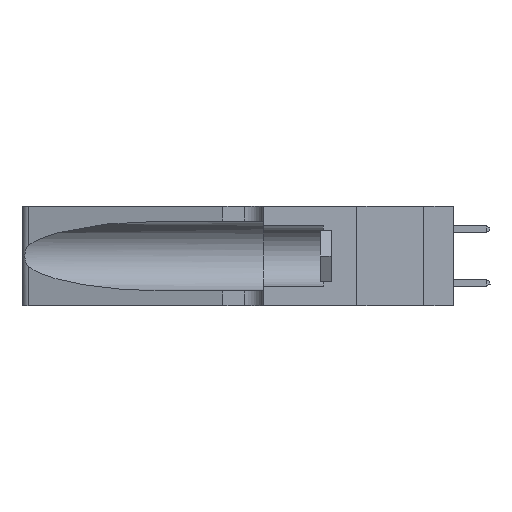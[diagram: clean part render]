
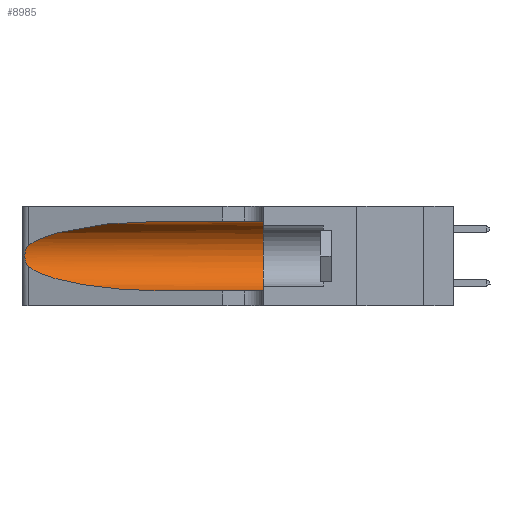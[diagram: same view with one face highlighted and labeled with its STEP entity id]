
A CAD part, left-side view. The second image highlights one B-rep face of the part: STEP entity #8985.
In plain terms, the highlighted cylindrical face has radius 3.308 mm (diameter 6.617 mm), a partial arc.
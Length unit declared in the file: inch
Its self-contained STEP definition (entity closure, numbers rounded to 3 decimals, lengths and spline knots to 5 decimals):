
#34 = EDGE_CURVE ( 'NONE', #14676, #33107, #30316, .T. ) ;
#211 = CARTESIAN_POINT ( 'NONE',  ( 0.25639, 1.23184, 0.21858 ) ) ;
#421 = CARTESIAN_POINT ( 'NONE',  ( 0.2373, 1.15595, 0.28018 ) ) ;
#486 = CARTESIAN_POINT ( 'NONE',  ( 0.25856, 1.23593, 0.16098 ) ) ;
#1070 = CARTESIAN_POINT ( 'NONE',  ( 0.25789, 1.23486, 0.15765 ) ) ;
#1306 = DIRECTION ( 'NONE',  ( 0., 0., -1. ) ) ;
#2062 = CARTESIAN_POINT ( 'NONE',  ( 0.25555, 1.22994, 0.2215 ) ) ;
#2919 = ORIENTED_EDGE ( 'NONE', *, *, #20586, .F. ) ;
#3013 = AXIS2_PLACEMENT_3D ( 'NONE', #5828, #29142, #30174 ) ;
#3647 = DIRECTION ( 'NONE',  ( 0., -1., 0. ) ) ;
#5679 = CARTESIAN_POINT ( 'NONE',  ( 0.1305, 0.72297, 0.31525 ) ) ;
#5828 = CARTESIAN_POINT ( 'NONE',  ( 0.1305, 0.35, 0.185 ) ) ;
#5906 = CARTESIAN_POINT ( 'NONE',  ( 0.25487, 1.22718, 0.22369 ) ) ;
#6838 = DIRECTION ( 'NONE',  ( 0., -1., 0. ) ) ;
#7635 = CARTESIAN_POINT ( 'NONE',  ( 0.26018, 1.23835, 0.19895 ) ) ;
#8394 =( BOUNDED_CURVE ( )  B_SPLINE_CURVE ( 3, ( #21341, #16261, #421, #5906 ),
 .UNSPECIFIED., .F., .F. ) 
 B_SPLINE_CURVE_WITH_KNOTS ( ( 4, 4 ),
 ( 1.5708, 2.84003 ),
 .UNSPECIFIED. ) 
 CURVE ( )  GEOMETRIC_REPRESENTATION_ITEM ( )  RATIONAL_B_SPLINE_CURVE ( ( 1., 0.87, 0.87, 1. ) ) 
 REPRESENTATION_ITEM ( '' )  );
#8648 = CARTESIAN_POINT ( 'NONE',  ( 0.25487, 1.22718, 0.14631 ) ) ;
#8985 = ADVANCED_FACE ( 'NONE', ( #12718 ), #25996, .F. ) ;
#9529 = CARTESIAN_POINT ( 'NONE',  ( 0.25487, 1.22718, 0.14631 ) ) ;
#9655 = CARTESIAN_POINT ( 'NONE',  ( 0.2373, 1.15595, 0.08982 ) ) ;
#9683 = VERTEX_POINT ( 'NONE', #11235 ) ;
#9748 = VERTEX_POINT ( 'NONE', #22189 ) ;
#9838 = CARTESIAN_POINT ( 'NONE',  ( 0.1305, 0.72297, 0.05475 ) ) ;
#11102 = ORIENTED_EDGE ( 'NONE', *, *, #24218, .T. ) ;
#11235 = CARTESIAN_POINT ( 'NONE',  ( 0.1305, 0.35, 0.31525 ) ) ;
#11658 = LINE ( 'NONE', #23118, #17342 ) ;
#12718 = FACE_OUTER_BOUND ( 'NONE', #22485, .T. ) ;
#12796 = CARTESIAN_POINT ( 'NONE',  ( 0.26075, 1.23896, 0.19203 ) ) ;
#14385 =( BOUNDED_CURVE ( )  B_SPLINE_CURVE ( 3, ( #9529, #9655, #22608, #32643 ),
 .UNSPECIFIED., .F., .T. ) 
 B_SPLINE_CURVE_WITH_KNOTS ( ( 4, 4 ),
 ( 3.44316, 4.71239 ),
 .UNSPECIFIED. ) 
 CURVE ( )  GEOMETRIC_REPRESENTATION_ITEM ( )  RATIONAL_B_SPLINE_CURVE ( ( 1., 0.87, 0.87, 1. ) ) 
 REPRESENTATION_ITEM ( '' )  );
#14672 = EDGE_CURVE ( 'NONE', #9683, #9748, #23970, .T. ) ;
#14676 = VERTEX_POINT ( 'NONE', #20736 ) ;
#15828 = CARTESIAN_POINT ( 'NONE',  ( 0.25854, 1.2359, 0.20912 ) ) ;
#16261 = CARTESIAN_POINT ( 'NONE',  ( 0.18966, 0.96281, 0.31525 ) ) ;
#16985 = CARTESIAN_POINT ( 'NONE',  ( 0.25487, 1.22718, 0.22369 ) ) ;
#17342 = VECTOR ( 'NONE', #17824, 39.37008 ) ;
#17824 = DIRECTION ( 'NONE',  ( 0., -1., 0. ) ) ;
#17952 = EDGE_CURVE ( 'NONE', #33107, #20655, #14385, .T. ) ;
#18443 = VERTEX_POINT ( 'NONE', #5679 ) ;
#19013 = ORIENTED_EDGE ( 'NONE', *, *, #14672, .F. ) ;
#19266 = ORIENTED_EDGE ( 'NONE', *, *, #31913, .T. ) ;
#19477 = CARTESIAN_POINT ( 'NONE',  ( 0.25487, 1.22718, 0.14631 ) ) ;
#20097 = ORIENTED_EDGE ( 'NONE', *, *, #34, .T. ) ;
#20586 = EDGE_CURVE ( 'NONE', #18443, #9683, #11658, .T. ) ;
#20655 = VERTEX_POINT ( 'NONE', #9838 ) ;
#20736 = CARTESIAN_POINT ( 'NONE',  ( 0.25487, 1.22718, 0.22369 ) ) ;
#21341 = CARTESIAN_POINT ( 'NONE',  ( 0.1305, 0.72297, 0.31525 ) ) ;
#21412 = LINE ( 'NONE', #32761, #28251 ) ;
#22130 = CARTESIAN_POINT ( 'NONE',  ( 0.25639, 1.23186, 0.15144 ) ) ;
#22189 = CARTESIAN_POINT ( 'NONE',  ( 0.1305, 0.35, 0.05475 ) ) ;
#22485 = EDGE_LOOP ( 'NONE', ( #11102, #20097, #26004, #19266, #19013, #2919 ) ) ;
#22608 = CARTESIAN_POINT ( 'NONE',  ( 0.18966, 0.96281, 0.05475 ) ) ;
#23118 = CARTESIAN_POINT ( 'NONE',  ( 0.1305, 1.61858, 0.31525 ) ) ;
#23486 = CARTESIAN_POINT ( 'NONE',  ( 0.25787, 1.23484, 0.2124 ) ) ;
#23970 = CIRCLE ( 'NONE', #3013, 0.13025 ) ;
#24170 = AXIS2_PLACEMENT_3D ( 'NONE', #24318, #3647, #1306 ) ;
#24218 = EDGE_CURVE ( 'NONE', #18443, #14676, #8394, .T. ) ;
#24318 = CARTESIAN_POINT ( 'NONE',  ( 0.1305, 1.61858, 0.185 ) ) ;
#25996 = CYLINDRICAL_SURFACE ( 'NONE', #24170, 0.13025 ) ;
#26004 = ORIENTED_EDGE ( 'NONE', *, *, #17952, .T. ) ;
#26534 = CARTESIAN_POINT ( 'NONE',  ( 0.25555, 1.22993, 0.14849 ) ) ;
#28251 = VECTOR ( 'NONE', #6838, 39.37008 ) ;
#29142 = DIRECTION ( 'NONE',  ( 0., 1., 0. ) ) ;
#30174 = DIRECTION ( 'NONE',  ( 0., 0., 1. ) ) ;
#30316 = B_SPLINE_CURVE_WITH_KNOTS ( 'NONE', 3,
 ( #16985, #2062, #211, #23486, #15828, #7635, #12796, #30819, #31677, #486, #1070, #22130, #26534, #8648 ),
 .UNSPECIFIED., .F., .F.,
 ( 4, 2, 2, 2, 2, 2, 4 ),
 ( 0., 0.00027, 0.00053, 0.00107, 0.0016, 0.00187, 0.00214 ),
 .UNSPECIFIED. ) ;
#30819 = CARTESIAN_POINT ( 'NONE',  ( 0.26075, 1.23896, 0.178 ) ) ;
#31677 = CARTESIAN_POINT ( 'NONE',  ( 0.26017, 1.23833, 0.17102 ) ) ;
#31913 = EDGE_CURVE ( 'NONE', #20655, #9748, #21412, .T. ) ;
#32643 = CARTESIAN_POINT ( 'NONE',  ( 0.1305, 0.72297, 0.05475 ) ) ;
#32761 = CARTESIAN_POINT ( 'NONE',  ( 0.1305, 1.61858, 0.05475 ) ) ;
#33107 = VERTEX_POINT ( 'NONE', #19477 ) ;
